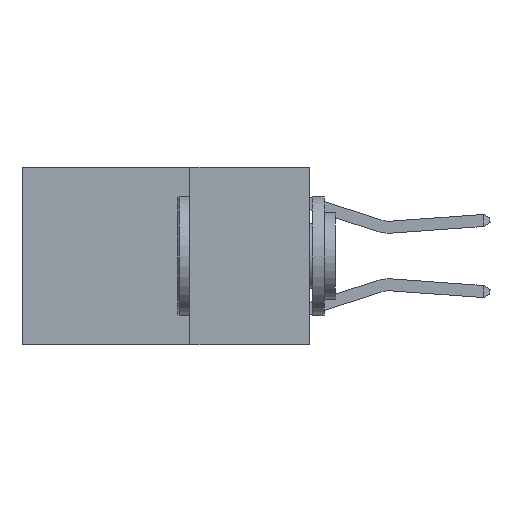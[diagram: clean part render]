
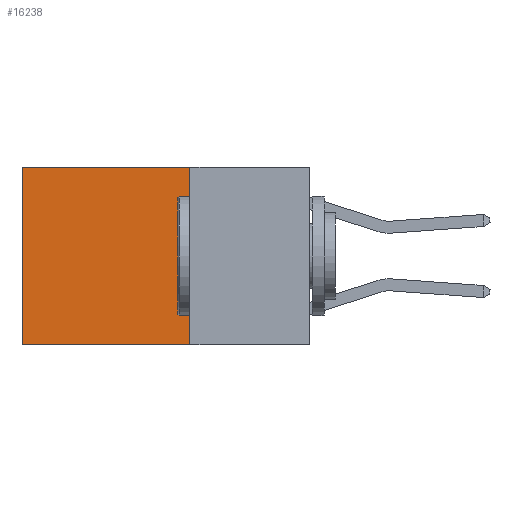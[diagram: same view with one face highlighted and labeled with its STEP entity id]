
A CAD part, left-side view. The second image highlights one B-rep face of the part: STEP entity #16238.
In plain terms, the highlighted planar face has unit normal (-1, 0, 0).
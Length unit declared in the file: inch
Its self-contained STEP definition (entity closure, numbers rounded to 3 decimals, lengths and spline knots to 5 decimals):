
#62 = VECTOR ( 'NONE', #8203, 39.37008 ) ;
#169 = CARTESIAN_POINT ( 'NONE',  ( 0.2625, 0.25, -0.37 ) ) ;
#477 = CARTESIAN_POINT ( 'NONE',  ( 0.2625, 0.6, 0. ) ) ;
#849 = VERTEX_POINT ( 'NONE', #14876 ) ;
#1014 = DIRECTION ( 'NONE',  ( 0., 0., -1. ) ) ;
#1058 = VECTOR ( 'NONE', #1014, 39.37008 ) ;
#1358 = LINE ( 'NONE', #3957, #1058 ) ;
#1479 = VERTEX_POINT ( 'NONE', #15742 ) ;
#1741 = EDGE_CURVE ( 'NONE', #5527, #1479, #13728, .T. ) ;
#2098 = ORIENTED_EDGE ( 'NONE', *, *, #9109, .F. ) ;
#3049 = LINE ( 'NONE', #14828, #62 ) ;
#3136 = CARTESIAN_POINT ( 'NONE',  ( 0.2625, 0.6, 0. ) ) ;
#3856 = VECTOR ( 'NONE', #11112, 39.37008 ) ;
#3957 = CARTESIAN_POINT ( 'NONE',  ( 0.2625, 0.25, 0. ) ) ;
#4514 = VERTEX_POINT ( 'NONE', #169 ) ;
#5527 = VERTEX_POINT ( 'NONE', #3136 ) ;
#6228 = EDGE_CURVE ( 'NONE', #849, #5527, #12508, .T. ) ;
#6476 = FACE_OUTER_BOUND ( 'NONE', #6672, .T. ) ;
#6672 = EDGE_LOOP ( 'NONE', ( #16914, #15981, #2098, #7873 ) ) ;
#7143 = DIRECTION ( 'NONE',  ( 1., 0., 0. ) ) ;
#7873 = ORIENTED_EDGE ( 'NONE', *, *, #6228, .T. ) ;
#8203 = DIRECTION ( 'NONE',  ( 0., 1., 0. ) ) ;
#8552 = CARTESIAN_POINT ( 'NONE',  ( 0.2625, 0.25, 0. ) ) ;
#9109 = EDGE_CURVE ( 'NONE', #849, #4514, #1358, .T. ) ;
#9609 = VECTOR ( 'NONE', #15124, 39.37008 ) ;
#9943 = DIRECTION ( 'NONE',  ( 0., 0., -1. ) ) ;
#10215 = PLANE ( 'NONE',  #14509 ) ;
#11112 = DIRECTION ( 'NONE',  ( 0., 1., 0. ) ) ;
#11357 = CARTESIAN_POINT ( 'NONE',  ( 0.2625, 0.25, 0. ) ) ;
#12508 = LINE ( 'NONE', #11357, #3856 ) ;
#13728 = LINE ( 'NONE', #477, #9609 ) ;
#14509 = AXIS2_PLACEMENT_3D ( 'NONE', #8552, #7143, #9943 ) ;
#14828 = CARTESIAN_POINT ( 'NONE',  ( 0.2625, 0.25, -0.37 ) ) ;
#14876 = CARTESIAN_POINT ( 'NONE',  ( 0.2625, 0.25, 0. ) ) ;
#15124 = DIRECTION ( 'NONE',  ( 0., 0., -1. ) ) ;
#15742 = CARTESIAN_POINT ( 'NONE',  ( 0.2625, 0.6, -0.37 ) ) ;
#15981 = ORIENTED_EDGE ( 'NONE', *, *, #16599, .F. ) ;
#16238 = ADVANCED_FACE ( 'NONE', ( #6476 ), #10215, .F. ) ;
#16599 = EDGE_CURVE ( 'NONE', #4514, #1479, #3049, .T. ) ;
#16914 = ORIENTED_EDGE ( 'NONE', *, *, #1741, .T. ) ;
